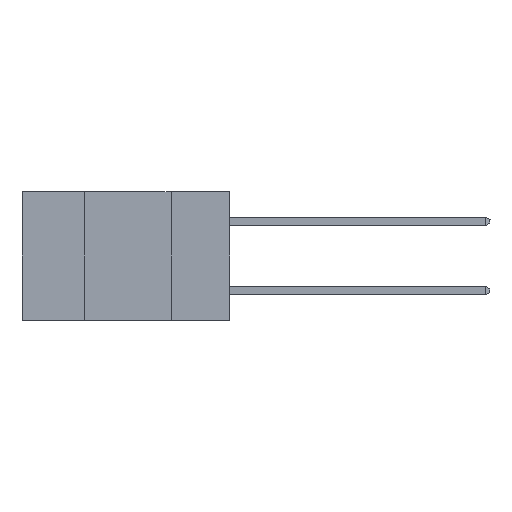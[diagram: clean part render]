
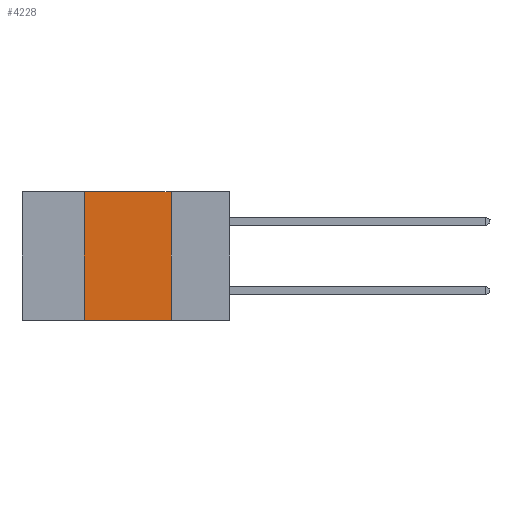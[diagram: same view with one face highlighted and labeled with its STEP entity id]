
A CAD part, left-side view. The second image highlights one B-rep face of the part: STEP entity #4228.
In plain terms, the highlighted planar face has unit normal (-1, 0, 0).
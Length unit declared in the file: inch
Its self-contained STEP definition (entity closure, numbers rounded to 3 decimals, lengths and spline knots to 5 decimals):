
#571 = PLANE ( 'NONE',  #1835 ) ;
#886 = DIRECTION ( 'NONE',  ( 0., 0., -1. ) ) ;
#1264 = LINE ( 'NONE', #5606, #7190 ) ;
#1775 = ORIENTED_EDGE ( 'NONE', *, *, #11343, .F. ) ;
#1835 = AXIS2_PLACEMENT_3D ( 'NONE', #12857, #12905, #13066 ) ;
#3113 = DIRECTION ( 'NONE',  ( 0., -1., 0. ) ) ;
#3119 = VERTEX_POINT ( 'NONE', #10448 ) ;
#3330 = EDGE_CURVE ( 'NONE', #3119, #10116, #11008, .T. ) ;
#3865 = ORIENTED_EDGE ( 'NONE', *, *, #3330, .F. ) ;
#4228 = ADVANCED_FACE ( 'NONE', ( #5982 ), #571, .F. ) ;
#4580 = VECTOR ( 'NONE', #886, 39.37008 ) ;
#5606 = CARTESIAN_POINT ( 'NONE',  ( 0., 0.6, 0. ) ) ;
#5806 = EDGE_CURVE ( 'NONE', #3119, #12845, #9063, .T. ) ;
#5982 = FACE_OUTER_BOUND ( 'NONE', #10717, .T. ) ;
#6371 = VECTOR ( 'NONE', #6915, 39.37008 ) ;
#6915 = DIRECTION ( 'NONE',  ( 0., -1., 0. ) ) ;
#7100 = LINE ( 'NONE', #13228, #4580 ) ;
#7190 = VECTOR ( 'NONE', #3113, 39.37008 ) ;
#7351 = EDGE_CURVE ( 'NONE', #8195, #12845, #7100, .T. ) ;
#8195 = VERTEX_POINT ( 'NONE', #15406 ) ;
#8443 = CARTESIAN_POINT ( 'NONE',  ( 0., 0.42, 0. ) ) ;
#8609 = CARTESIAN_POINT ( 'NONE',  ( 0., 0.42, 0. ) ) ;
#9063 = LINE ( 'NONE', #11958, #6371 ) ;
#10116 = VERTEX_POINT ( 'NONE', #8609 ) ;
#10367 = CARTESIAN_POINT ( 'NONE',  ( 0., 0.17, -0.37 ) ) ;
#10442 = ORIENTED_EDGE ( 'NONE', *, *, #5806, .T. ) ;
#10448 = CARTESIAN_POINT ( 'NONE',  ( 0., 0.42, -0.37 ) ) ;
#10717 = EDGE_LOOP ( 'NONE', ( #15798, #1775, #3865, #10442 ) ) ;
#10871 = DIRECTION ( 'NONE',  ( 0., 0., 1. ) ) ;
#11008 = LINE ( 'NONE', #8443, #12343 ) ;
#11343 = EDGE_CURVE ( 'NONE', #10116, #8195, #1264, .T. ) ;
#11958 = CARTESIAN_POINT ( 'NONE',  ( 0., 0.6, -0.37 ) ) ;
#12343 = VECTOR ( 'NONE', #10871, 39.37008 ) ;
#12845 = VERTEX_POINT ( 'NONE', #10367 ) ;
#12857 = CARTESIAN_POINT ( 'NONE',  ( 0., 0.6, 0. ) ) ;
#12905 = DIRECTION ( 'NONE',  ( 1., 0., 0. ) ) ;
#13066 = DIRECTION ( 'NONE',  ( 0., 0., -1. ) ) ;
#13228 = CARTESIAN_POINT ( 'NONE',  ( 0., 0.17, 0. ) ) ;
#15406 = CARTESIAN_POINT ( 'NONE',  ( 0., 0.17, 0. ) ) ;
#15798 = ORIENTED_EDGE ( 'NONE', *, *, #7351, .F. ) ;
